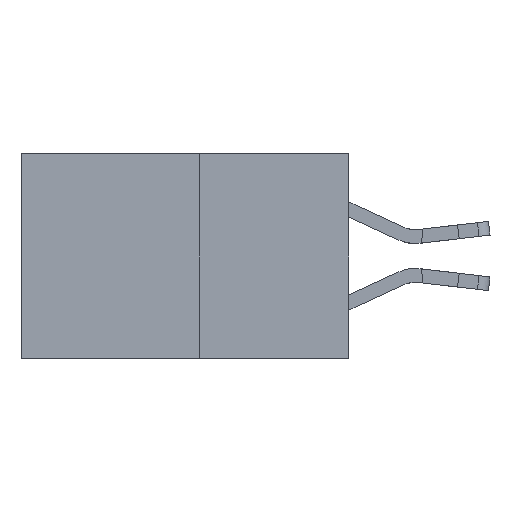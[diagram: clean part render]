
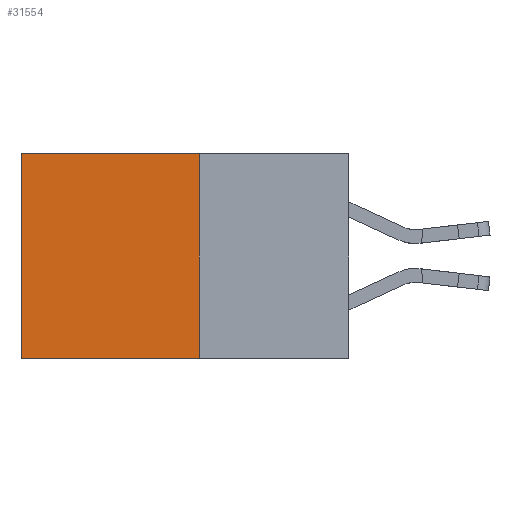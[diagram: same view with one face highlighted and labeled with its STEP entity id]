
A CAD part, left-side view. The second image highlights one B-rep face of the part: STEP entity #31554.
In plain terms, the highlighted planar face has unit normal (-1, 0, 0).
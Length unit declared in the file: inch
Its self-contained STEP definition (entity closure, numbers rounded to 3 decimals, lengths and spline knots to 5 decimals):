
#391 = DIRECTION ( 'NONE',  ( 0., 0., -1. ) ) ;
#1143 = VERTEX_POINT ( 'NONE', #11131 ) ;
#1173 = DIRECTION ( 'NONE',  ( 0., 0., -1. ) ) ;
#1565 = DIRECTION ( 'NONE',  ( 0., 0., -1. ) ) ;
#2219 = LINE ( 'NONE', #4542, #14738 ) ;
#2967 = ORIENTED_EDGE ( 'NONE', *, *, #24976, .T. ) ;
#3014 = LINE ( 'NONE', #30103, #21261 ) ;
#3090 = VERTEX_POINT ( 'NONE', #24109 ) ;
#4055 = ORIENTED_EDGE ( 'NONE', *, *, #15854, .T. ) ;
#4096 = FACE_OUTER_BOUND ( 'NONE', #23569, .T. ) ;
#4542 = CARTESIAN_POINT ( 'NONE',  ( 0.277, 0.27, 0. ) ) ;
#6084 = VERTEX_POINT ( 'NONE', #21847 ) ;
#7018 = DIRECTION ( 'NONE',  ( 0., 1., 0. ) ) ;
#9552 = VECTOR ( 'NONE', #1565, 39.37008 ) ;
#11131 = CARTESIAN_POINT ( 'NONE',  ( 0.277, 0.59, -0.37 ) ) ;
#11502 = EDGE_CURVE ( 'NONE', #23911, #6084, #21421, .T. ) ;
#12986 = DIRECTION ( 'NONE',  ( 0., 1., 0. ) ) ;
#14738 = VECTOR ( 'NONE', #7018, 39.37008 ) ;
#15321 = DIRECTION ( 'NONE',  ( 1., 0., 0. ) ) ;
#15854 = EDGE_CURVE ( 'NONE', #3090, #1143, #17029, .T. ) ;
#17029 = LINE ( 'NONE', #31097, #9552 ) ;
#18611 = CARTESIAN_POINT ( 'NONE',  ( 0.277, 0.27, -0.37 ) ) ;
#20008 = ORIENTED_EDGE ( 'NONE', *, *, #24542, .F. ) ;
#20748 = AXIS2_PLACEMENT_3D ( 'NONE', #29951, #15321, #391 ) ;
#21261 = VECTOR ( 'NONE', #12986, 39.37008 ) ;
#21421 = LINE ( 'NONE', #18611, #27183 ) ;
#21847 = CARTESIAN_POINT ( 'NONE',  ( 0.277, 0.27, -0.37 ) ) ;
#23569 = EDGE_LOOP ( 'NONE', ( #4055, #20008, #28558, #2967 ) ) ;
#23911 = VERTEX_POINT ( 'NONE', #27510 ) ;
#24109 = CARTESIAN_POINT ( 'NONE',  ( 0.277, 0.59, 0. ) ) ;
#24542 = EDGE_CURVE ( 'NONE', #6084, #1143, #3014, .T. ) ;
#24976 = EDGE_CURVE ( 'NONE', #23911, #3090, #2219, .T. ) ;
#27183 = VECTOR ( 'NONE', #1173, 39.37008 ) ;
#27510 = CARTESIAN_POINT ( 'NONE',  ( 0.277, 0.27, 0. ) ) ;
#27525 = PLANE ( 'NONE',  #20748 ) ;
#28558 = ORIENTED_EDGE ( 'NONE', *, *, #11502, .F. ) ;
#29951 = CARTESIAN_POINT ( 'NONE',  ( 0.277, 0.27, -0.37 ) ) ;
#30103 = CARTESIAN_POINT ( 'NONE',  ( 0.277, 0.27, -0.37 ) ) ;
#31097 = CARTESIAN_POINT ( 'NONE',  ( 0.277, 0.59, -0.37 ) ) ;
#31554 = ADVANCED_FACE ( 'NONE', ( #4096 ), #27525, .F. ) ;
